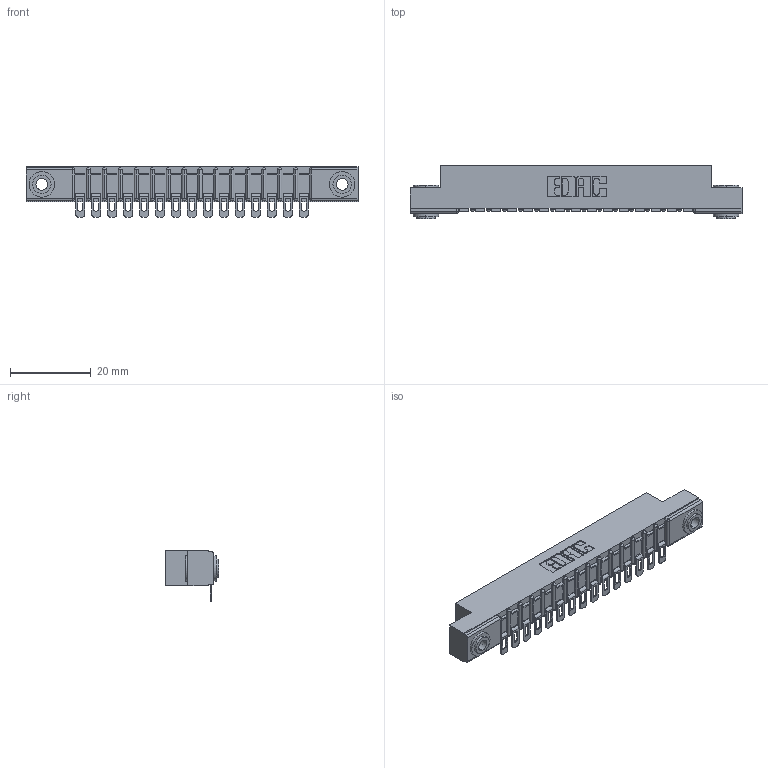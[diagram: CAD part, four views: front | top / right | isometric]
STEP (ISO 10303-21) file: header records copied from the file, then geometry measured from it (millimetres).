
FILE_DESCRIPTION (( 'STEP AP203' ), '1' );
FILE_NAME ('357-015-554-103.STEP', '2019-09-16T20:25:24', ( '' ), ( '' ), 'SwSTEP 2.0', 'SolidWorks 2016', '' );
FILE_SCHEMA (( 'CONFIG_CONTROL_DESIGN' ));
Length unit declared in the file: inch
Products named in the file (4): 345-250-002_345-250-002-102; 357-015-554-103; 307-290-002_554; 307 Part_.156 Dia Mounting Holes
Assembly tree (18 placements, depth 2):
  357-015-554-103
    307 Part_.156 Dia Mounting Holes
    307-290-002_554  x15
    345-250-002_345-250-002-102  x2
Bounding box: 82.45 x 13.36 x 12.52 mm (x, y, z)
Volume: 5446.1 mm3; surface area: 9822 mm2
Topology: 18 solids, 18 shells, 1401 faces, 4230 edges, 2772 vertices
Faces by surface type: plane 784, cylinder 577, sphere 32, cone 8
Entity records: 18218 total; most frequent: CARTESIAN_POINT 3047, ORIENTED_EDGE 3028, DIRECTION 2994, EDGE_CURVE 1514, LINE 1132, VECTOR 1132, VERTEX_POINT 984, AXIS2_PLACEMENT_3D 931
